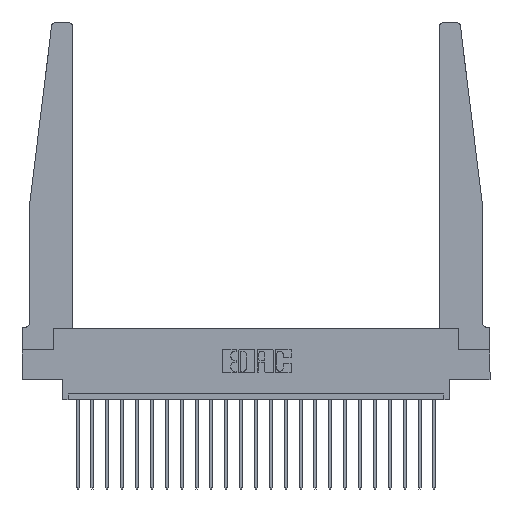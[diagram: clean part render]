
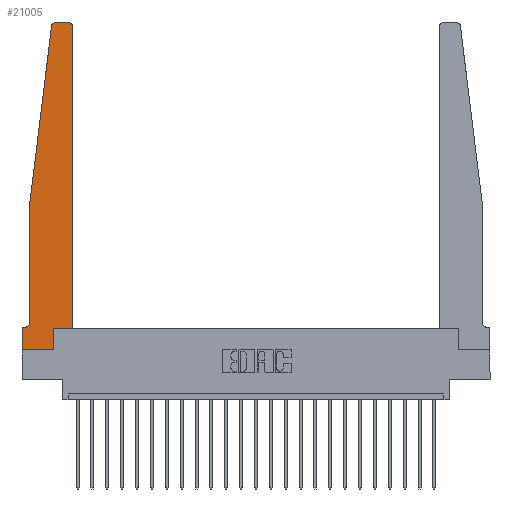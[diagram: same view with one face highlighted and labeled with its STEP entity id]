
A CAD part, top view. The second image highlights one B-rep face of the part: STEP entity #21005.
In plain terms, the highlighted planar face has unit normal (0, 0, 1).
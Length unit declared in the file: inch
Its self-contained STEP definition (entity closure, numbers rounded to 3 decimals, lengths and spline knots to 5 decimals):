
#9 = CIRCLE ( 'NONE', #11429, 0.03 ) ;
#43 = ORIENTED_EDGE ( 'NONE', *, *, #241, .T. ) ;
#59 = VERTEX_POINT ( 'NONE', #4884 ) ;
#96 = CARTESIAN_POINT ( 'NONE',  ( 0.425, 2.72, 0.37 ) ) ;
#129 = VERTEX_POINT ( 'NONE', #2448 ) ;
#151 = LINE ( 'NONE', #8500, #18227 ) ;
#225 = VECTOR ( 'NONE', #13003, 39.37008 ) ;
#241 = EDGE_CURVE ( 'NONE', #10434, #13803, #21393, .T. ) ;
#296 = FACE_OUTER_BOUND ( 'NONE', #19694, .T. ) ;
#748 = LINE ( 'NONE', #20314, #225 ) ;
#1203 = CARTESIAN_POINT ( 'NONE',  ( 0.015, 0.2375, 0.37 ) ) ;
#1275 = DIRECTION ( 'NONE',  ( 0., 0., -1. ) ) ;
#1553 = DIRECTION ( 'NONE',  ( 1., 0., 0. ) ) ;
#1804 = DIRECTION ( 'NONE',  ( -1., 0., 0. ) ) ;
#2181 = CARTESIAN_POINT ( 'NONE',  ( 0.065, 0.1875, 0.37 ) ) ;
#2195 = ORIENTED_EDGE ( 'NONE', *, *, #17679, .T. ) ;
#2448 = CARTESIAN_POINT ( 'NONE',  ( 0.065, 1.25, 0.37 ) ) ;
#2518 = VERTEX_POINT ( 'NONE', #6708 ) ;
#2582 = EDGE_CURVE ( 'NONE', #10455, #129, #12983, .T. ) ;
#3077 = VERTEX_POINT ( 'NONE', #20345 ) ;
#3198 = CIRCLE ( 'NONE', #6494, 0.03 ) ;
#3357 = CARTESIAN_POINT ( 'NONE',  ( 0.425, 0.18, 0.37 ) ) ;
#3562 = VERTEX_POINT ( 'NONE', #16575 ) ;
#3959 = EDGE_CURVE ( 'NONE', #129, #2518, #11277, .T. ) ;
#4085 = ORIENTED_EDGE ( 'NONE', *, *, #20629, .T. ) ;
#4498 = CARTESIAN_POINT ( 'NONE',  ( 0.395, 2.72, 0.37 ) ) ;
#4578 = ORIENTED_EDGE ( 'NONE', *, *, #3959, .T. ) ;
#4884 = CARTESIAN_POINT ( 'NONE',  ( 0.2605, 0.18, 0.37 ) ) ;
#5573 = EDGE_CURVE ( 'NONE', #6769, #3077, #9, .T. ) ;
#6103 = ORIENTED_EDGE ( 'NONE', *, *, #9375, .T. ) ;
#6321 = DIRECTION ( 'NONE',  ( 0., -1., 0. ) ) ;
#6378 = ORIENTED_EDGE ( 'NONE', *, *, #5573, .T. ) ;
#6494 = AXIS2_PLACEMENT_3D ( 'NONE', #13799, #19476, #10561 ) ;
#6694 = DIRECTION ( 'NONE',  ( 0., 1., 0. ) ) ;
#6708 = CARTESIAN_POINT ( 'NONE',  ( 0.065, 0.2375, 0.37 ) ) ;
#6769 = VERTEX_POINT ( 'NONE', #96 ) ;
#7029 = ORIENTED_EDGE ( 'NONE', *, *, #2582, .T. ) ;
#7047 = ORIENTED_EDGE ( 'NONE', *, *, #12902, .T. ) ;
#7092 = CARTESIAN_POINT ( 'NONE',  ( 0., 0., 0.37 ) ) ;
#7103 = DIRECTION ( 'NONE',  ( -0.122, -0.992, 0. ) ) ;
#7422 = LINE ( 'NONE', #17021, #12350 ) ;
#7444 = AXIS2_PLACEMENT_3D ( 'NONE', #1203, #1275, #16876 ) ;
#8500 = CARTESIAN_POINT ( 'NONE',  ( 0.425, 0.18, 0.37 ) ) ;
#9136 = DIRECTION ( 'NONE',  ( -1., 0., 0. ) ) ;
#9375 = EDGE_CURVE ( 'NONE', #22738, #6769, #151, .T. ) ;
#9845 = CARTESIAN_POINT ( 'NONE',  ( 0., 0., 0.37 ) ) ;
#10434 = VERTEX_POINT ( 'NONE', #17215 ) ;
#10455 = VERTEX_POINT ( 'NONE', #16996 ) ;
#10459 = CARTESIAN_POINT ( 'NONE',  ( 0.27653, 2.75, 0.37 ) ) ;
#10539 = LINE ( 'NONE', #3357, #21580 ) ;
#10561 = DIRECTION ( 'NONE',  ( 1., 0., 0. ) ) ;
#11277 = LINE ( 'NONE', #12160, #16533 ) ;
#11429 = AXIS2_PLACEMENT_3D ( 'NONE', #4498, #11580, #13315 ) ;
#11477 = LINE ( 'NONE', #20964, #16719 ) ;
#11580 = DIRECTION ( 'NONE',  ( 0., 0., 1. ) ) ;
#11647 = CARTESIAN_POINT ( 'NONE',  ( 0.425, 0.18, 0.37 ) ) ;
#11649 = VECTOR ( 'NONE', #7103, 39.37008 ) ;
#12160 = CARTESIAN_POINT ( 'NONE',  ( 0.065, 1.25, 0.37 ) ) ;
#12350 = VECTOR ( 'NONE', #18761, 39.37008 ) ;
#12598 = VECTOR ( 'NONE', #9136, 39.37008 ) ;
#12902 = EDGE_CURVE ( 'NONE', #13700, #10455, #3198, .T. ) ;
#12912 = EDGE_CURVE ( 'NONE', #20736, #10434, #17504, .T. ) ;
#12983 = LINE ( 'NONE', #14076, #11649 ) ;
#13003 = DIRECTION ( 'NONE',  ( 0., 1., 0. ) ) ;
#13315 = DIRECTION ( 'NONE',  ( 1., 0., 0. ) ) ;
#13489 = ORIENTED_EDGE ( 'NONE', *, *, #12912, .T. ) ;
#13700 = VERTEX_POINT ( 'NONE', #10459 ) ;
#13799 = CARTESIAN_POINT ( 'NONE',  ( 0.27653, 2.72, 0.37 ) ) ;
#13803 = VERTEX_POINT ( 'NONE', #7092 ) ;
#14070 = EDGE_CURVE ( 'NONE', #2518, #20736, #15856, .T. ) ;
#14076 = CARTESIAN_POINT ( 'NONE',  ( 0.065, 1.25, 0.37 ) ) ;
#14198 = VECTOR ( 'NONE', #6321, 39.37008 ) ;
#14234 = ORIENTED_EDGE ( 'NONE', *, *, #14070, .T. ) ;
#14603 = PLANE ( 'NONE',  #21083 ) ;
#14823 = CARTESIAN_POINT ( 'NONE',  ( 0., 0.1875, 0.37 ) ) ;
#15639 = EDGE_CURVE ( 'NONE', #3077, #13700, #11477, .T. ) ;
#15856 = CIRCLE ( 'NONE', #7444, 0.05 ) ;
#16324 = DIRECTION ( 'NONE',  ( 1., 0., 0. ) ) ;
#16471 = DIRECTION ( 'NONE',  ( 0., 0., 1. ) ) ;
#16533 = VECTOR ( 'NONE', #19353, 39.37008 ) ;
#16575 = CARTESIAN_POINT ( 'NONE',  ( 0.2605, 0., 0.37 ) ) ;
#16719 = VECTOR ( 'NONE', #1804, 39.37008 ) ;
#16876 = DIRECTION ( 'NONE',  ( -1., 0., 0. ) ) ;
#16996 = CARTESIAN_POINT ( 'NONE',  ( 0.24675, 2.72367, 0.37 ) ) ;
#17021 = CARTESIAN_POINT ( 'NONE',  ( 0., 0., 0.37 ) ) ;
#17215 = CARTESIAN_POINT ( 'NONE',  ( 0., 0.1875, 0.37 ) ) ;
#17322 = CARTESIAN_POINT ( 'NONE',  ( 0.015, 0.1875, 0.37 ) ) ;
#17504 = LINE ( 'NONE', #2181, #12598 ) ;
#17679 = EDGE_CURVE ( 'NONE', #59, #22738, #10539, .T. ) ;
#18227 = VECTOR ( 'NONE', #6694, 39.37008 ) ;
#18761 = DIRECTION ( 'NONE',  ( 1., 0., 0. ) ) ;
#19353 = DIRECTION ( 'NONE',  ( 0., -1., 0. ) ) ;
#19476 = DIRECTION ( 'NONE',  ( 0., 0., 1. ) ) ;
#19694 = EDGE_LOOP ( 'NONE', ( #21205, #7047, #7029, #4578, #14234, #13489, #43, #4085, #20357, #2195, #6103, #6378 ) ) ;
#20314 = CARTESIAN_POINT ( 'NONE',  ( 0.2605, 0.18, 0.37 ) ) ;
#20345 = CARTESIAN_POINT ( 'NONE',  ( 0.395, 2.75, 0.37 ) ) ;
#20357 = ORIENTED_EDGE ( 'NONE', *, *, #22676, .T. ) ;
#20629 = EDGE_CURVE ( 'NONE', #13803, #3562, #7422, .T. ) ;
#20736 = VERTEX_POINT ( 'NONE', #17322 ) ;
#20964 = CARTESIAN_POINT ( 'NONE',  ( 0.25, 2.75, 0.37 ) ) ;
#21005 = ADVANCED_FACE ( 'NONE', ( #296 ), #14603, .T. ) ;
#21083 = AXIS2_PLACEMENT_3D ( 'NONE', #14823, #16471, #16324 ) ;
#21205 = ORIENTED_EDGE ( 'NONE', *, *, #15639, .T. ) ;
#21393 = LINE ( 'NONE', #9845, #14198 ) ;
#21580 = VECTOR ( 'NONE', #1553, 39.37008 ) ;
#22676 = EDGE_CURVE ( 'NONE', #3562, #59, #748, .T. ) ;
#22738 = VERTEX_POINT ( 'NONE', #11647 ) ;
